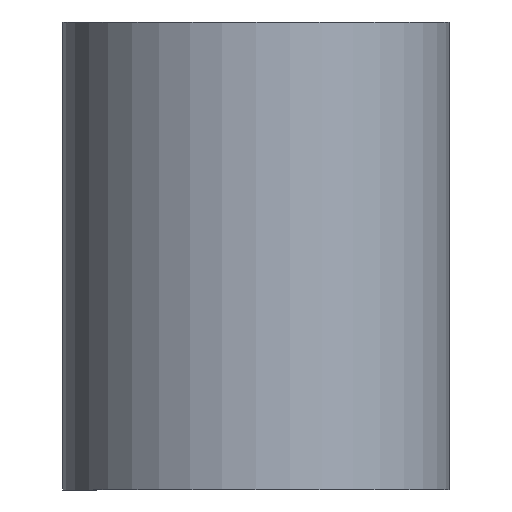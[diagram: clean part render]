
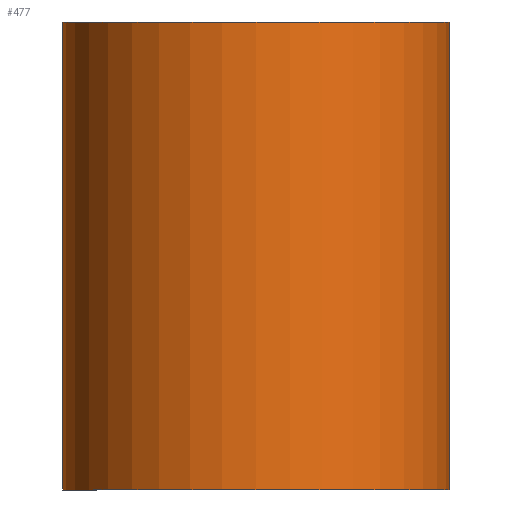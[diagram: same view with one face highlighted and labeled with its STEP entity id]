
A CAD part, front view. The second image highlights one B-rep face of the part: STEP entity #477.
In plain terms, the highlighted cylindrical face has radius 18.567 mm (diameter 37.133 mm), a partial arc.
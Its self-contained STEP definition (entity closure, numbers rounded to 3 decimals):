
#45 = VECTOR ( 'NONE', #665, 1000. ) ;
#53 = EDGE_CURVE ( 'NONE', #1434, #1415, #351, .T. ) ;
#105 = ORIENTED_EDGE ( 'NONE', *, *, #53, .F. ) ;
#183 = CARTESIAN_POINT ( 'NONE',  ( -171.598, -88.078, -22.488 ) ) ;
#199 = ORIENTED_EDGE ( 'NONE', *, *, #1263, .T. ) ;
#201 = ORIENTED_EDGE ( 'NONE', *, *, #1209, .T. ) ;
#250 = LINE ( 'NONE', #660, #45 ) ;
#340 = AXIS2_PLACEMENT_3D ( 'NONE', #451, #447, #446 ) ;
#344 = VECTOR ( 'NONE', #1206, 1000. ) ;
#351 = LINE ( 'NONE', #1218, #344 ) ;
#446 = DIRECTION ( 'NONE',  ( 1., 0., 0. ) ) ;
#447 = DIRECTION ( 'NONE',  ( 0., 0., 1. ) ) ;
#451 = CARTESIAN_POINT ( 'NONE',  ( -190.165, -88.078, 22.512 ) ) ;
#473 = AXIS2_PLACEMENT_3D ( 'NONE', #721, #718, #717 ) ;
#477 = ADVANCED_FACE ( 'NONE', ( #686 ), #671, .T. ) ;
#486 = CARTESIAN_POINT ( 'NONE',  ( -208.731, -88.078, -22.488 ) ) ;
#495 = CARTESIAN_POINT ( 'NONE',  ( -208.731, -88.078, 22.512 ) ) ;
#660 = CARTESIAN_POINT ( 'NONE',  ( -171.598, -88.078, -22.488 ) ) ;
#665 = DIRECTION ( 'NONE',  ( 0., 0., 1. ) ) ;
#671 = CYLINDRICAL_SURFACE ( 'NONE', #828, 18.567 ) ;
#686 = FACE_OUTER_BOUND ( 'NONE', #778, .T. ) ;
#717 = DIRECTION ( 'NONE',  ( 1., 0., 0. ) ) ;
#718 = DIRECTION ( 'NONE',  ( 0., 0., 1. ) ) ;
#721 = CARTESIAN_POINT ( 'NONE',  ( -190.165, -88.078, -22.488 ) ) ;
#778 = EDGE_LOOP ( 'NONE', ( #833, #105, #201, #199 ) ) ;
#828 = AXIS2_PLACEMENT_3D ( 'NONE', #1058, #1055, #1059 ) ;
#833 = ORIENTED_EDGE ( 'NONE', *, *, #1439, .F. ) ;
#1055 = DIRECTION ( 'NONE',  ( 0., 0., 1. ) ) ;
#1058 = CARTESIAN_POINT ( 'NONE',  ( -190.165, -88.078, -22.488 ) ) ;
#1059 = DIRECTION ( 'NONE',  ( 1., 0., 0. ) ) ;
#1206 = DIRECTION ( 'NONE',  ( 0., 0., 1. ) ) ;
#1209 = EDGE_CURVE ( 'NONE', #1434, #1575, #1484, .T. ) ;
#1218 = CARTESIAN_POINT ( 'NONE',  ( -208.731, -88.078, -22.488 ) ) ;
#1263 = EDGE_CURVE ( 'NONE', #1575, #1421, #250, .T. ) ;
#1388 = CIRCLE ( 'NONE', #340, 18.567 ) ;
#1415 = VERTEX_POINT ( 'NONE', #495 ) ;
#1421 = VERTEX_POINT ( 'NONE', #1599 ) ;
#1434 = VERTEX_POINT ( 'NONE', #486 ) ;
#1439 = EDGE_CURVE ( 'NONE', #1415, #1421, #1388, .T. ) ;
#1484 = CIRCLE ( 'NONE', #473, 18.567 ) ;
#1575 = VERTEX_POINT ( 'NONE', #183 ) ;
#1599 = CARTESIAN_POINT ( 'NONE',  ( -171.598, -88.078, 22.512 ) ) ;
